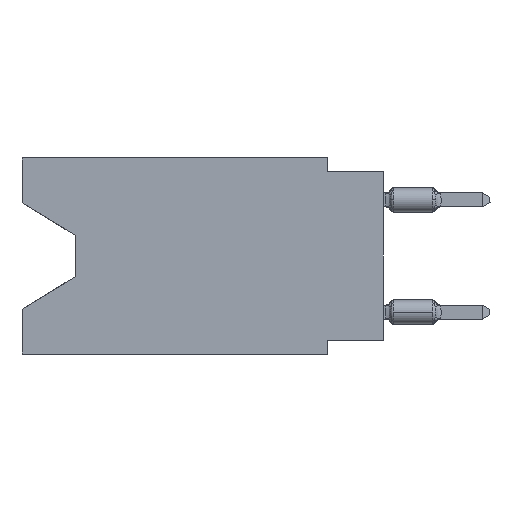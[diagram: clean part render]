
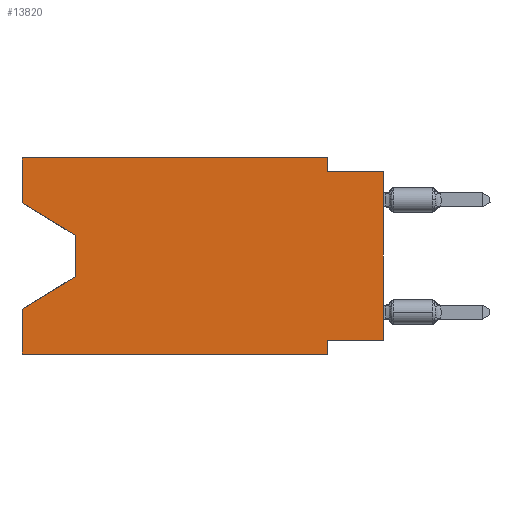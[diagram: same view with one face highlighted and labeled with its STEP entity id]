
A CAD part, left-side view. The second image highlights one B-rep face of the part: STEP entity #13820.
In plain terms, the highlighted planar face has unit normal (-1, 0, 0).
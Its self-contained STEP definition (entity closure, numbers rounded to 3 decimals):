
#93 = LINE ( 'NONE', #7724, #13143 ) ;
#226 = DIRECTION ( 'NONE',  ( 0., 0., 1. ) ) ;
#386 = CARTESIAN_POINT ( 'NONE',  ( 0., 16.383, 0. ) ) ;
#390 = LINE ( 'NONE', #13745, #15308 ) ;
#474 = ORIENTED_EDGE ( 'NONE', *, *, #22474, .T. ) ;
#645 = VERTEX_POINT ( 'NONE', #19905 ) ;
#829 = VECTOR ( 'NONE', #20712, 1000. ) ;
#1042 = DIRECTION ( 'NONE',  ( 0., 1., 0. ) ) ;
#1281 = VERTEX_POINT ( 'NONE', #15605 ) ;
#1284 = LINE ( 'NONE', #18156, #15139 ) ;
#1518 = ORIENTED_EDGE ( 'NONE', *, *, #15631, .F. ) ;
#1620 = VECTOR ( 'NONE', #22367, 1000. ) ;
#1883 = VECTOR ( 'NONE', #13682, 1000. ) ;
#2019 = VECTOR ( 'NONE', #17433, 1000. ) ;
#2140 = FACE_OUTER_BOUND ( 'NONE', #15724, .T. ) ;
#2579 = EDGE_CURVE ( 'NONE', #645, #15511, #16214, .T. ) ;
#2894 = VERTEX_POINT ( 'NONE', #22956 ) ;
#3004 = CARTESIAN_POINT ( 'NONE',  ( 0., 0., -0.635 ) ) ;
#3965 = CARTESIAN_POINT ( 'NONE',  ( 0., 13.97, -5.385 ) ) ;
#4017 = CARTESIAN_POINT ( 'NONE',  ( 0., 16.383, -6.852 ) ) ;
#4105 = CARTESIAN_POINT ( 'NONE',  ( 0., 2.54, 0. ) ) ;
#4319 = LINE ( 'NONE', #15436, #2019 ) ;
#4714 = EDGE_CURVE ( 'NONE', #21811, #2894, #1284, .T. ) ;
#4860 = CARTESIAN_POINT ( 'NONE',  ( 0., 2.54, -8.89 ) ) ;
#5027 = VERTEX_POINT ( 'NONE', #12250 ) ;
#5379 = CARTESIAN_POINT ( 'NONE',  ( 0., 16.383, 0. ) ) ;
#5631 = DIRECTION ( 'NONE',  ( 0., 0., -1. ) ) ;
#5694 = ORIENTED_EDGE ( 'NONE', *, *, #2579, .T. ) ;
#5833 = CARTESIAN_POINT ( 'NONE',  ( 0., 13.97, -5.385 ) ) ;
#6218 = LINE ( 'NONE', #4105, #23691 ) ;
#6375 = EDGE_CURVE ( 'NONE', #20905, #5027, #12989, .T. ) ;
#6381 = ORIENTED_EDGE ( 'NONE', *, *, #24454, .T. ) ;
#6886 = DIRECTION ( 'NONE',  ( 0., -1., 0. ) ) ;
#7112 = LINE ( 'NONE', #14728, #1620 ) ;
#7724 = CARTESIAN_POINT ( 'NONE',  ( 0., 16.383, 0. ) ) ;
#8192 = LINE ( 'NONE', #23064, #1883 ) ;
#8466 = CARTESIAN_POINT ( 'NONE',  ( 0., 16.383, 0. ) ) ;
#9000 = EDGE_CURVE ( 'NONE', #21811, #9253, #11031, .T. ) ;
#9062 = VECTOR ( 'NONE', #9157, 1000. ) ;
#9157 = DIRECTION ( 'NONE',  ( 0., 0., 1. ) ) ;
#9253 = VERTEX_POINT ( 'NONE', #3004 ) ;
#9475 = CARTESIAN_POINT ( 'NONE',  ( 0., 13.97, -3.505 ) ) ;
#9706 = LINE ( 'NONE', #5833, #829 ) ;
#10008 = VECTOR ( 'NONE', #6886, 1000. ) ;
#10223 = DIRECTION ( 'NONE',  ( 0., -0.855, -0.519 ) ) ;
#11031 = LINE ( 'NONE', #20907, #9062 ) ;
#11413 = LINE ( 'NONE', #17157, #23922 ) ;
#11507 = EDGE_CURVE ( 'NONE', #645, #20905, #93, .T. ) ;
#11845 = EDGE_CURVE ( 'NONE', #15511, #24496, #4319, .T. ) ;
#12190 = ORIENTED_EDGE ( 'NONE', *, *, #21614, .F. ) ;
#12250 = CARTESIAN_POINT ( 'NONE',  ( 0., 2.54, 0. ) ) ;
#12989 = LINE ( 'NONE', #5379, #10008 ) ;
#13143 = VECTOR ( 'NONE', #226, 1000. ) ;
#13172 = ORIENTED_EDGE ( 'NONE', *, *, #6375, .F. ) ;
#13681 = VECTOR ( 'NONE', #10223, 1000. ) ;
#13682 = DIRECTION ( 'NONE',  ( 0., -1., 0. ) ) ;
#13717 = VERTEX_POINT ( 'NONE', #16498 ) ;
#13745 = CARTESIAN_POINT ( 'NONE',  ( 0., 2.54, -8.89 ) ) ;
#13820 = ADVANCED_FACE ( 'NONE', ( #2140 ), #15501, .F. ) ;
#13955 = DIRECTION ( 'NONE',  ( 0., 0., -1. ) ) ;
#14728 = CARTESIAN_POINT ( 'NONE',  ( 0., 16.383, -8.89 ) ) ;
#15114 = EDGE_CURVE ( 'NONE', #2894, #15401, #390, .T. ) ;
#15139 = VECTOR ( 'NONE', #1042, 1000. ) ;
#15308 = VECTOR ( 'NONE', #19140, 1000. ) ;
#15401 = VERTEX_POINT ( 'NONE', #4860 ) ;
#15436 = CARTESIAN_POINT ( 'NONE',  ( 0., 13.97, -3.505 ) ) ;
#15501 = PLANE ( 'NONE',  #22692 ) ;
#15511 = VERTEX_POINT ( 'NONE', #9475 ) ;
#15605 = CARTESIAN_POINT ( 'NONE',  ( 0., 2.54, -0.635 ) ) ;
#15631 = EDGE_CURVE ( 'NONE', #5027, #1281, #6218, .T. ) ;
#15724 = EDGE_LOOP ( 'NONE', ( #5694, #24631, #6381, #12190, #474, #19748, #20888, #23684, #19755, #1518, #13172, #18613 ) ) ;
#16214 = LINE ( 'NONE', #21729, #13681 ) ;
#16498 = CARTESIAN_POINT ( 'NONE',  ( 0., 16.383, -8.89 ) ) ;
#17157 = CARTESIAN_POINT ( 'NONE',  ( 0., 16.383, 0. ) ) ;
#17433 = DIRECTION ( 'NONE',  ( 0., 0., -1. ) ) ;
#18156 = CARTESIAN_POINT ( 'NONE',  ( 0., 0., -8.255 ) ) ;
#18613 = ORIENTED_EDGE ( 'NONE', *, *, #11507, .F. ) ;
#19140 = DIRECTION ( 'NONE',  ( 0., 0., -1. ) ) ;
#19286 = VERTEX_POINT ( 'NONE', #4017 ) ;
#19748 = ORIENTED_EDGE ( 'NONE', *, *, #15114, .F. ) ;
#19755 = ORIENTED_EDGE ( 'NONE', *, *, #20151, .F. ) ;
#19905 = CARTESIAN_POINT ( 'NONE',  ( 0., 16.383, -2.038 ) ) ;
#20151 = EDGE_CURVE ( 'NONE', #1281, #9253, #8192, .T. ) ;
#20712 = DIRECTION ( 'NONE',  ( 0., 0.855, -0.519 ) ) ;
#20888 = ORIENTED_EDGE ( 'NONE', *, *, #4714, .F. ) ;
#20905 = VERTEX_POINT ( 'NONE', #8466 ) ;
#20907 = CARTESIAN_POINT ( 'NONE',  ( 0., 0., 0. ) ) ;
#21013 = DIRECTION ( 'NONE',  ( 1., 0., 0. ) ) ;
#21049 = DIRECTION ( 'NONE',  ( 0., 0., 1. ) ) ;
#21614 = EDGE_CURVE ( 'NONE', #13717, #19286, #11413, .T. ) ;
#21655 = CARTESIAN_POINT ( 'NONE',  ( 0., 0., -8.255 ) ) ;
#21729 = CARTESIAN_POINT ( 'NONE',  ( 0., 16.383, -2.038 ) ) ;
#21811 = VERTEX_POINT ( 'NONE', #21655 ) ;
#22367 = DIRECTION ( 'NONE',  ( 0., -1., 0. ) ) ;
#22474 = EDGE_CURVE ( 'NONE', #13717, #15401, #7112, .T. ) ;
#22692 = AXIS2_PLACEMENT_3D ( 'NONE', #386, #21013, #5631 ) ;
#22956 = CARTESIAN_POINT ( 'NONE',  ( 0., 2.54, -8.255 ) ) ;
#23064 = CARTESIAN_POINT ( 'NONE',  ( 0., 0., -0.635 ) ) ;
#23684 = ORIENTED_EDGE ( 'NONE', *, *, #9000, .T. ) ;
#23691 = VECTOR ( 'NONE', #13955, 1000. ) ;
#23922 = VECTOR ( 'NONE', #21049, 1000. ) ;
#24454 = EDGE_CURVE ( 'NONE', #24496, #19286, #9706, .T. ) ;
#24496 = VERTEX_POINT ( 'NONE', #3965 ) ;
#24631 = ORIENTED_EDGE ( 'NONE', *, *, #11845, .T. ) ;
